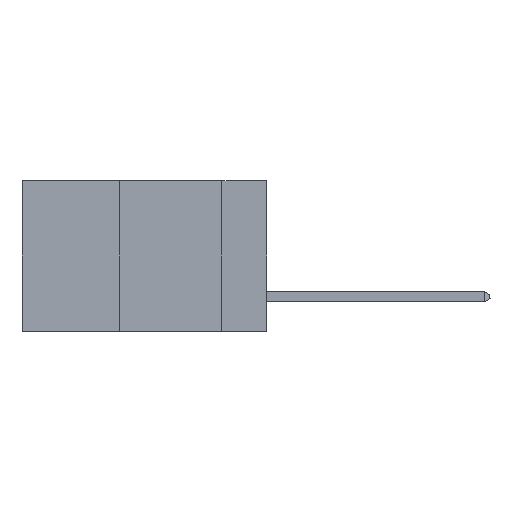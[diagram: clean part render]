
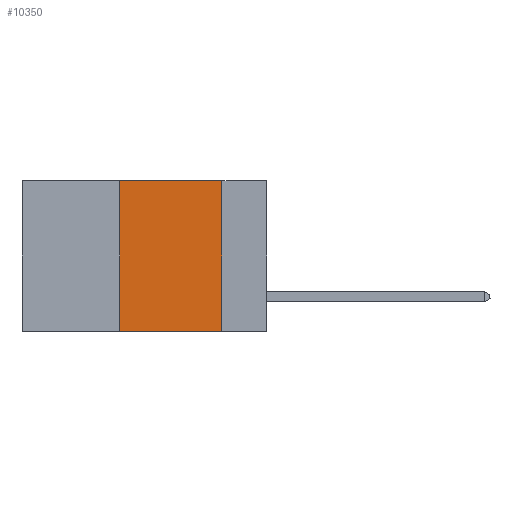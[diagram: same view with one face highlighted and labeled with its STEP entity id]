
A CAD part, left-side view. The second image highlights one B-rep face of the part: STEP entity #10350.
In plain terms, the highlighted planar face has unit normal (-1, 0, 0).
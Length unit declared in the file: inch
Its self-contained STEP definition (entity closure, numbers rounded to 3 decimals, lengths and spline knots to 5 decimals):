
#259 = LINE ( 'NONE', #7572, #683 ) ;
#532 = EDGE_CURVE ( 'NONE', #6428, #5841, #9890, .T. ) ;
#683 = VECTOR ( 'NONE', #1293, 39.37008 ) ;
#737 = VECTOR ( 'NONE', #3750, 39.37008 ) ;
#919 = AXIS2_PLACEMENT_3D ( 'NONE', #3001, #6606, #4955 ) ;
#1286 = EDGE_LOOP ( 'NONE', ( #10070, #7771, #6364, #10749 ) ) ;
#1293 = DIRECTION ( 'NONE',  ( 0., 0., -1. ) ) ;
#1917 = VECTOR ( 'NONE', #4141, 39.37008 ) ;
#3001 = CARTESIAN_POINT ( 'NONE',  ( 0., 0.6, 0. ) ) ;
#3108 = FACE_OUTER_BOUND ( 'NONE', #1286, .T. ) ;
#3750 = DIRECTION ( 'NONE',  ( 0., -1., 0. ) ) ;
#4028 = DIRECTION ( 'NONE',  ( 0., -1., 0. ) ) ;
#4141 = DIRECTION ( 'NONE',  ( 0., 0., 1. ) ) ;
#4644 = CARTESIAN_POINT ( 'NONE',  ( 0., 0.36, -0.37 ) ) ;
#4758 = EDGE_CURVE ( 'NONE', #6428, #7671, #8036, .T. ) ;
#4840 = PLANE ( 'NONE',  #919 ) ;
#4955 = DIRECTION ( 'NONE',  ( 0., 0., -1. ) ) ;
#5479 = LINE ( 'NONE', #7570, #6572 ) ;
#5841 = VERTEX_POINT ( 'NONE', #6553 ) ;
#6364 = ORIENTED_EDGE ( 'NONE', *, *, #532, .F. ) ;
#6428 = VERTEX_POINT ( 'NONE', #4644 ) ;
#6553 = CARTESIAN_POINT ( 'NONE',  ( 0., 0.36, 0. ) ) ;
#6572 = VECTOR ( 'NONE', #4028, 39.37008 ) ;
#6606 = DIRECTION ( 'NONE',  ( 1., 0., 0. ) ) ;
#6655 = CARTESIAN_POINT ( 'NONE',  ( 0., 0.11, 0. ) ) ;
#6743 = CARTESIAN_POINT ( 'NONE',  ( 0., 0.36, 0. ) ) ;
#7570 = CARTESIAN_POINT ( 'NONE',  ( 0., 0.6, 0. ) ) ;
#7572 = CARTESIAN_POINT ( 'NONE',  ( 0., 0.11, 0. ) ) ;
#7671 = VERTEX_POINT ( 'NONE', #10566 ) ;
#7771 = ORIENTED_EDGE ( 'NONE', *, *, #10308, .F. ) ;
#8036 = LINE ( 'NONE', #8042, #737 ) ;
#8042 = CARTESIAN_POINT ( 'NONE',  ( 0., 0.6, -0.37 ) ) ;
#8470 = EDGE_CURVE ( 'NONE', #9835, #7671, #259, .T. ) ;
#9835 = VERTEX_POINT ( 'NONE', #6655 ) ;
#9890 = LINE ( 'NONE', #6743, #1917 ) ;
#10070 = ORIENTED_EDGE ( 'NONE', *, *, #8470, .F. ) ;
#10308 = EDGE_CURVE ( 'NONE', #5841, #9835, #5479, .T. ) ;
#10350 = ADVANCED_FACE ( 'NONE', ( #3108 ), #4840, .F. ) ;
#10566 = CARTESIAN_POINT ( 'NONE',  ( 0., 0.11, -0.37 ) ) ;
#10749 = ORIENTED_EDGE ( 'NONE', *, *, #4758, .T. ) ;
